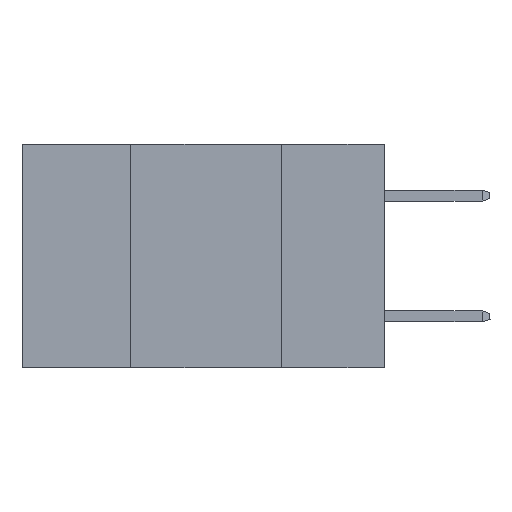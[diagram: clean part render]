
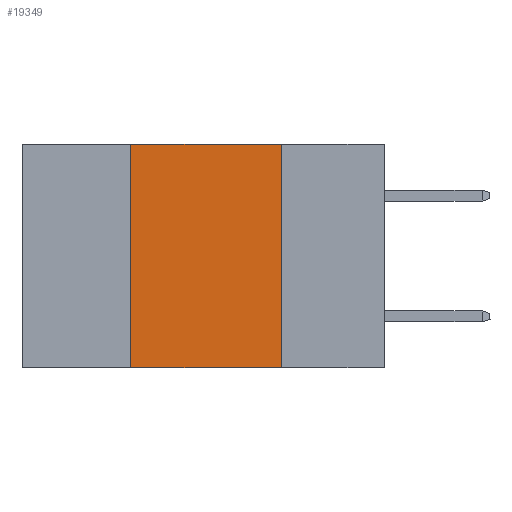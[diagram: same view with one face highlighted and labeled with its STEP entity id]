
A CAD part, left-side view. The second image highlights one B-rep face of the part: STEP entity #19349.
In plain terms, the highlighted planar face has unit normal (-1, 0, 0).
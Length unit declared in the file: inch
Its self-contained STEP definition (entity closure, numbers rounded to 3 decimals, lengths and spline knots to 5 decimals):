
#225 = VECTOR ( 'NONE', #4756, 39.37008 ) ;
#858 = CARTESIAN_POINT ( 'NONE',  ( 0., 0.17, -0.37 ) ) ;
#2726 = EDGE_CURVE ( 'NONE', #10553, #18845, #7421, .T. ) ;
#2864 = CARTESIAN_POINT ( 'NONE',  ( 0., 0.17, 0. ) ) ;
#4756 = DIRECTION ( 'NONE',  ( 0., 0., -1. ) ) ;
#5101 = VECTOR ( 'NONE', #11702, 39.37008 ) ;
#6387 = ORIENTED_EDGE ( 'NONE', *, *, #16064, .F. ) ;
#7087 = VERTEX_POINT ( 'NONE', #18049 ) ;
#7421 = LINE ( 'NONE', #23053, #26264 ) ;
#7695 = LINE ( 'NONE', #2864, #225 ) ;
#8985 = DIRECTION ( 'NONE',  ( 0., 0., -1. ) ) ;
#9086 = CARTESIAN_POINT ( 'NONE',  ( 0., 0.6, 0. ) ) ;
#9242 = VERTEX_POINT ( 'NONE', #9294 ) ;
#9294 = CARTESIAN_POINT ( 'NONE',  ( 0., 0.17, 0. ) ) ;
#9310 = EDGE_CURVE ( 'NONE', #9242, #18845, #7695, .T. ) ;
#9454 = DIRECTION ( 'NONE',  ( 0., -1., 0. ) ) ;
#9707 = ORIENTED_EDGE ( 'NONE', *, *, #2726, .T. ) ;
#9839 = CARTESIAN_POINT ( 'NONE',  ( 0., 0.42, -0.37 ) ) ;
#10553 = VERTEX_POINT ( 'NONE', #9839 ) ;
#11702 = DIRECTION ( 'NONE',  ( 0., -1., 0. ) ) ;
#12162 = VECTOR ( 'NONE', #22488, 39.37008 ) ;
#13063 = AXIS2_PLACEMENT_3D ( 'NONE', #9086, #20236, #8985 ) ;
#13766 = PLANE ( 'NONE',  #13063 ) ;
#14204 = EDGE_CURVE ( 'NONE', #10553, #7087, #15343, .T. ) ;
#15086 = ORIENTED_EDGE ( 'NONE', *, *, #9310, .F. ) ;
#15343 = LINE ( 'NONE', #22386, #12162 ) ;
#16064 = EDGE_CURVE ( 'NONE', #7087, #9242, #29278, .T. ) ;
#18049 = CARTESIAN_POINT ( 'NONE',  ( 0., 0.42, 0. ) ) ;
#18373 = CARTESIAN_POINT ( 'NONE',  ( 0., 0.6, 0. ) ) ;
#18845 = VERTEX_POINT ( 'NONE', #858 ) ;
#19349 = ADVANCED_FACE ( 'NONE', ( #24828 ), #13766, .F. ) ;
#20236 = DIRECTION ( 'NONE',  ( 1., 0., 0. ) ) ;
#21751 = ORIENTED_EDGE ( 'NONE', *, *, #14204, .F. ) ;
#22062 = EDGE_LOOP ( 'NONE', ( #15086, #6387, #21751, #9707 ) ) ;
#22386 = CARTESIAN_POINT ( 'NONE',  ( 0., 0.42, 0. ) ) ;
#22488 = DIRECTION ( 'NONE',  ( 0., 0., 1. ) ) ;
#23053 = CARTESIAN_POINT ( 'NONE',  ( 0., 0.6, -0.37 ) ) ;
#24828 = FACE_OUTER_BOUND ( 'NONE', #22062, .T. ) ;
#26264 = VECTOR ( 'NONE', #9454, 39.37008 ) ;
#29278 = LINE ( 'NONE', #18373, #5101 ) ;
